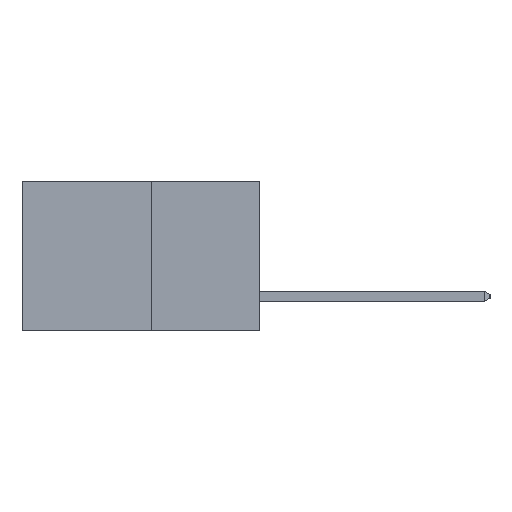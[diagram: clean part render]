
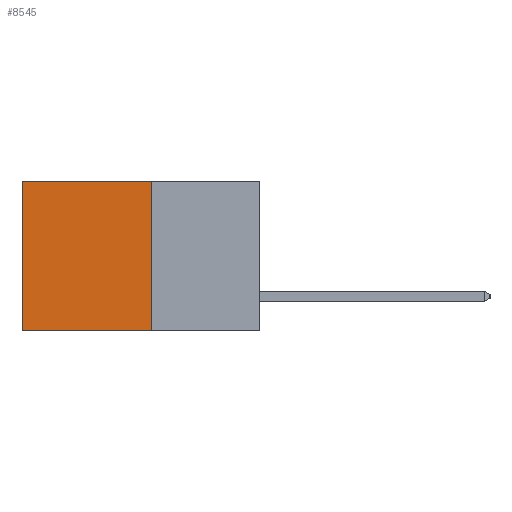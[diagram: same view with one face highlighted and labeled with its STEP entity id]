
A CAD part, left-side view. The second image highlights one B-rep face of the part: STEP entity #8545.
In plain terms, the highlighted planar face has unit normal (-1, 0, 0).
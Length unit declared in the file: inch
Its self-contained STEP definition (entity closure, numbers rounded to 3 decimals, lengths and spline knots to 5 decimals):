
#389 = DIRECTION ( 'NONE',  ( 0., 0., -1. ) ) ;
#572 = DIRECTION ( 'NONE',  ( 1., 0., 0. ) ) ;
#1079 = VERTEX_POINT ( 'NONE', #13126 ) ;
#1194 = LINE ( 'NONE', #7065, #9984 ) ;
#1653 = CARTESIAN_POINT ( 'NONE',  ( 0.277, 0.27, -0.37 ) ) ;
#1671 = DIRECTION ( 'NONE',  ( 0., 1., 0. ) ) ;
#1694 = VECTOR ( 'NONE', #389, 39.37008 ) ;
#1862 = ORIENTED_EDGE ( 'NONE', *, *, #4938, .F. ) ;
#2356 = ORIENTED_EDGE ( 'NONE', *, *, #7320, .T. ) ;
#2858 = ORIENTED_EDGE ( 'NONE', *, *, #7418, .F. ) ;
#4938 = EDGE_CURVE ( 'NONE', #1079, #11580, #7449, .T. ) ;
#5555 = AXIS2_PLACEMENT_3D ( 'NONE', #7202, #572, #8309 ) ;
#5661 = CARTESIAN_POINT ( 'NONE',  ( 0.277, 0.59, 0. ) ) ;
#6308 = EDGE_CURVE ( 'NONE', #8058, #6472, #1194, .T. ) ;
#6390 = CARTESIAN_POINT ( 'NONE',  ( 0.277, 0.59, -0.37 ) ) ;
#6472 = VERTEX_POINT ( 'NONE', #5661 ) ;
#6865 = LINE ( 'NONE', #10626, #9087 ) ;
#7065 = CARTESIAN_POINT ( 'NONE',  ( 0.277, 0.27, 0. ) ) ;
#7202 = CARTESIAN_POINT ( 'NONE',  ( 0.277, 0.27, -0.37 ) ) ;
#7320 = EDGE_CURVE ( 'NONE', #6472, #11580, #7545, .T. ) ;
#7418 = EDGE_CURVE ( 'NONE', #8058, #1079, #6865, .T. ) ;
#7449 = LINE ( 'NONE', #1653, #10373 ) ;
#7545 = LINE ( 'NONE', #8172, #1694 ) ;
#7593 = DIRECTION ( 'NONE',  ( 0., 1., 0. ) ) ;
#8058 = VERTEX_POINT ( 'NONE', #11871 ) ;
#8172 = CARTESIAN_POINT ( 'NONE',  ( 0.277, 0.59, -0.37 ) ) ;
#8309 = DIRECTION ( 'NONE',  ( 0., 0., -1. ) ) ;
#8545 = ADVANCED_FACE ( 'NONE', ( #12149 ), #13735, .F. ) ;
#9087 = VECTOR ( 'NONE', #12817, 39.37008 ) ;
#9984 = VECTOR ( 'NONE', #7593, 39.37008 ) ;
#10373 = VECTOR ( 'NONE', #1671, 39.37008 ) ;
#10626 = CARTESIAN_POINT ( 'NONE',  ( 0.277, 0.27, -0.37 ) ) ;
#10962 = EDGE_LOOP ( 'NONE', ( #2356, #1862, #2858, #11714 ) ) ;
#11580 = VERTEX_POINT ( 'NONE', #6390 ) ;
#11714 = ORIENTED_EDGE ( 'NONE', *, *, #6308, .T. ) ;
#11871 = CARTESIAN_POINT ( 'NONE',  ( 0.277, 0.27, 0. ) ) ;
#12149 = FACE_OUTER_BOUND ( 'NONE', #10962, .T. ) ;
#12817 = DIRECTION ( 'NONE',  ( 0., 0., -1. ) ) ;
#13126 = CARTESIAN_POINT ( 'NONE',  ( 0.277, 0.27, -0.37 ) ) ;
#13735 = PLANE ( 'NONE',  #5555 ) ;
